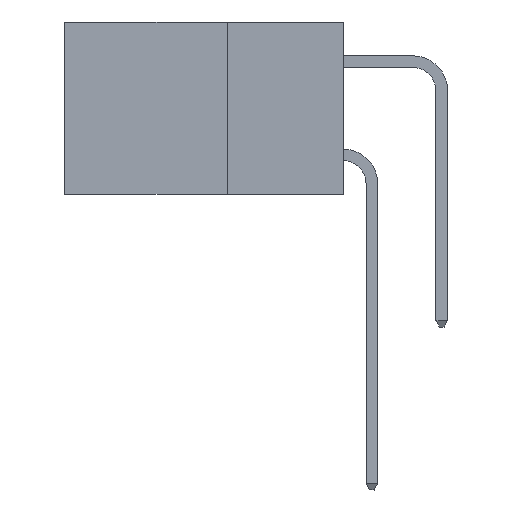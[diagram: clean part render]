
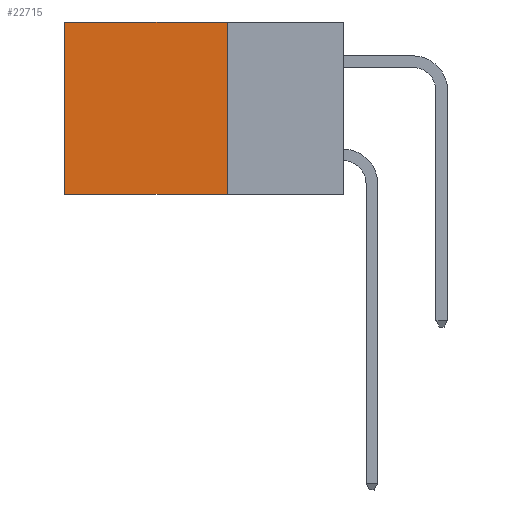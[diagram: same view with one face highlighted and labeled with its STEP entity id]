
A CAD part, left-side view. The second image highlights one B-rep face of the part: STEP entity #22715.
In plain terms, the highlighted planar face has unit normal (-1, 0, 0).
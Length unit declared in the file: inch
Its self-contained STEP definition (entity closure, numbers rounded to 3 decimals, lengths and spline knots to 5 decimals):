
#34 = VECTOR ( 'NONE', #7450, 39.37008 ) ;
#2151 = ORIENTED_EDGE ( 'NONE', *, *, #2726, .F. ) ;
#2726 = EDGE_CURVE ( 'NONE', #9693, #6342, #15189, .T. ) ;
#4452 = DIRECTION ( 'NONE',  ( 0., 1., 0. ) ) ;
#4464 = LINE ( 'NONE', #18131, #19048 ) ;
#6342 = VERTEX_POINT ( 'NONE', #8457 ) ;
#7450 = DIRECTION ( 'NONE',  ( 0., 0., -1. ) ) ;
#7800 = VERTEX_POINT ( 'NONE', #18307 ) ;
#7853 = DIRECTION ( 'NONE',  ( 0., 0., -1. ) ) ;
#8457 = CARTESIAN_POINT ( 'NONE',  ( 0.298, 0.6, -0.37 ) ) ;
#8895 = ORIENTED_EDGE ( 'NONE', *, *, #19798, .F. ) ;
#9485 = CARTESIAN_POINT ( 'NONE',  ( 0.298, 0.25, 0. ) ) ;
#9626 = LINE ( 'NONE', #16461, #34 ) ;
#9641 = DIRECTION ( 'NONE',  ( 0., 0., -1. ) ) ;
#9693 = VERTEX_POINT ( 'NONE', #16063 ) ;
#10442 = VERTEX_POINT ( 'NONE', #13102 ) ;
#10604 = EDGE_CURVE ( 'NONE', #10442, #6342, #9626, .T. ) ;
#11479 = PLANE ( 'NONE',  #13761 ) ;
#12157 = VECTOR ( 'NONE', #15888, 39.37008 ) ;
#13102 = CARTESIAN_POINT ( 'NONE',  ( 0.298, 0.6, 0. ) ) ;
#13761 = AXIS2_PLACEMENT_3D ( 'NONE', #18413, #20010, #7853 ) ;
#15189 = LINE ( 'NONE', #17745, #12157 ) ;
#15888 = DIRECTION ( 'NONE',  ( 0., 1., 0. ) ) ;
#16063 = CARTESIAN_POINT ( 'NONE',  ( 0.298, 0.25, -0.37 ) ) ;
#16187 = ORIENTED_EDGE ( 'NONE', *, *, #10604, .T. ) ;
#16401 = EDGE_LOOP ( 'NONE', ( #16187, #2151, #8895, #16723 ) ) ;
#16461 = CARTESIAN_POINT ( 'NONE',  ( 0.298, 0.6, 0. ) ) ;
#16723 = ORIENTED_EDGE ( 'NONE', *, *, #16867, .T. ) ;
#16867 = EDGE_CURVE ( 'NONE', #7800, #10442, #22078, .T. ) ;
#17745 = CARTESIAN_POINT ( 'NONE',  ( 0.298, 0.25, -0.37 ) ) ;
#18131 = CARTESIAN_POINT ( 'NONE',  ( 0.298, 0.25, 0. ) ) ;
#18307 = CARTESIAN_POINT ( 'NONE',  ( 0.298, 0.25, 0. ) ) ;
#18413 = CARTESIAN_POINT ( 'NONE',  ( 0.298, 0.25, 0. ) ) ;
#19048 = VECTOR ( 'NONE', #9641, 39.37008 ) ;
#19459 = FACE_OUTER_BOUND ( 'NONE', #16401, .T. ) ;
#19798 = EDGE_CURVE ( 'NONE', #7800, #9693, #4464, .T. ) ;
#20010 = DIRECTION ( 'NONE',  ( 1., 0., 0. ) ) ;
#22078 = LINE ( 'NONE', #9485, #22628 ) ;
#22628 = VECTOR ( 'NONE', #4452, 39.37008 ) ;
#22715 = ADVANCED_FACE ( 'NONE', ( #19459 ), #11479, .F. ) ;
